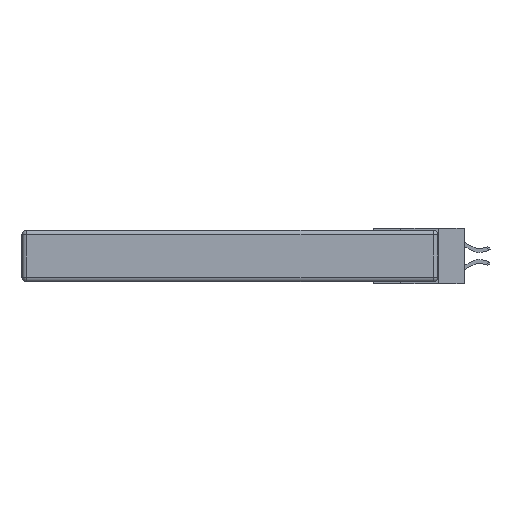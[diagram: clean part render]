
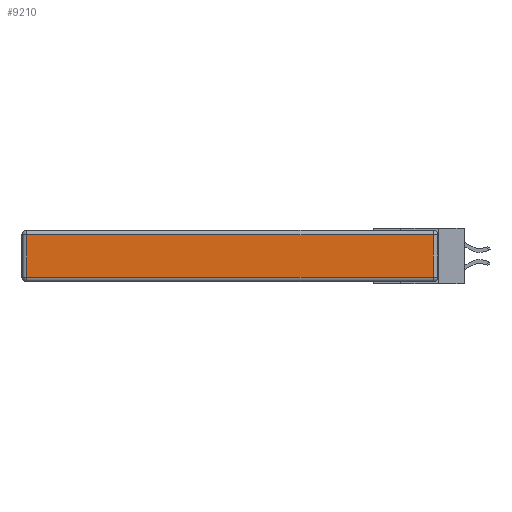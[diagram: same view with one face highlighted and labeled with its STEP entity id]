
A CAD part, left-side view. The second image highlights one B-rep face of the part: STEP entity #9210.
In plain terms, the highlighted planar face has unit normal (-1, 0, 0).
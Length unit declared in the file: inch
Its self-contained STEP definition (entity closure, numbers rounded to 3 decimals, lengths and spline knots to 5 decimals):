
#473 = ORIENTED_EDGE ( 'NONE', *, *, #6737, .T. ) ;
#789 = CARTESIAN_POINT ( 'NONE',  ( 0., 0.03, -0.03 ) ) ;
#2045 = CARTESIAN_POINT ( 'NONE',  ( 0., 2.72, -0.343 ) ) ;
#2298 = CARTESIAN_POINT ( 'NONE',  ( 0., 2.72, -0.313 ) ) ;
#3557 = VERTEX_POINT ( 'NONE', #4302 ) ;
#4302 = CARTESIAN_POINT ( 'NONE',  ( 0., 2.72, -0.03 ) ) ;
#5244 = LINE ( 'NONE', #2045, #31069 ) ;
#5892 = DIRECTION ( 'NONE',  ( 0., 0., 1. ) ) ;
#6176 = ORIENTED_EDGE ( 'NONE', *, *, #20319, .T. ) ;
#6737 = EDGE_CURVE ( 'NONE', #3557, #35241, #5244, .T. ) ;
#7062 = VERTEX_POINT ( 'NONE', #8985 ) ;
#7179 = VECTOR ( 'NONE', #5892, 39.37008 ) ;
#8390 = CARTESIAN_POINT ( 'NONE',  ( 0., 0., -0.343 ) ) ;
#8912 = CARTESIAN_POINT ( 'NONE',  ( 0., 0.03, -0.343 ) ) ;
#8985 = CARTESIAN_POINT ( 'NONE',  ( 0., 0.03, -0.313 ) ) ;
#9210 = ADVANCED_FACE ( 'NONE', ( #16780 ), #30040, .T. ) ;
#9336 = LINE ( 'NONE', #8912, #7179 ) ;
#10141 = DIRECTION ( 'NONE',  ( 0., 0., -1. ) ) ;
#10991 = CARTESIAN_POINT ( 'NONE',  ( 0., 2.75, -0.03 ) ) ;
#11106 = DIRECTION ( 'NONE',  ( 0., -1., 0. ) ) ;
#14972 = EDGE_LOOP ( 'NONE', ( #6176, #15873, #15519, #473 ) ) ;
#15037 = DIRECTION ( 'NONE',  ( 0., 0., 1. ) ) ;
#15519 = ORIENTED_EDGE ( 'NONE', *, *, #20202, .T. ) ;
#15612 = DIRECTION ( 'NONE',  ( -1., 0., 0. ) ) ;
#15873 = ORIENTED_EDGE ( 'NONE', *, *, #32417, .T. ) ;
#16383 = DIRECTION ( 'NONE',  ( 0., 1., 0. ) ) ;
#16508 = CARTESIAN_POINT ( 'NONE',  ( 0., 0., -0.313 ) ) ;
#16780 = FACE_OUTER_BOUND ( 'NONE', #14972, .T. ) ;
#17137 = VERTEX_POINT ( 'NONE', #789 ) ;
#20202 = EDGE_CURVE ( 'NONE', #17137, #3557, #27127, .T. ) ;
#20319 = EDGE_CURVE ( 'NONE', #35241, #7062, #21939, .T. ) ;
#21939 = LINE ( 'NONE', #16508, #24981 ) ;
#24099 = VECTOR ( 'NONE', #16383, 39.37008 ) ;
#24981 = VECTOR ( 'NONE', #11106, 39.37008 ) ;
#27127 = LINE ( 'NONE', #10991, #24099 ) ;
#30040 = PLANE ( 'NONE',  #30798 ) ;
#30798 = AXIS2_PLACEMENT_3D ( 'NONE', #8390, #15612, #15037 ) ;
#31069 = VECTOR ( 'NONE', #10141, 39.37008 ) ;
#32417 = EDGE_CURVE ( 'NONE', #7062, #17137, #9336, .T. ) ;
#35241 = VERTEX_POINT ( 'NONE', #2298 ) ;
